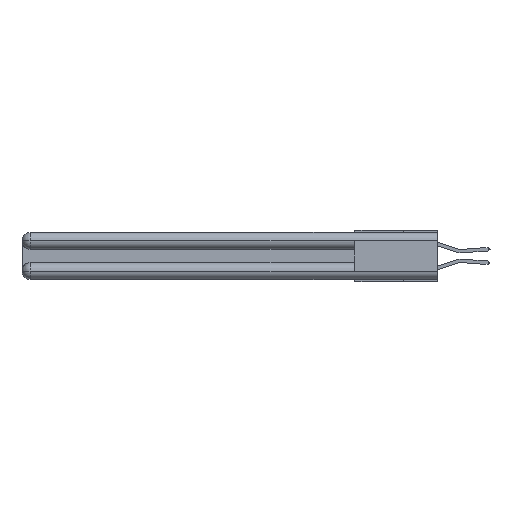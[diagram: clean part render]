
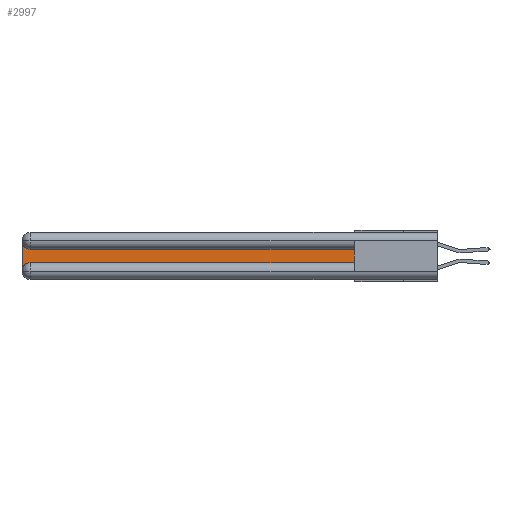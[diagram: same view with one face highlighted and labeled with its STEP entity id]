
A CAD part, left-side view. The second image highlights one B-rep face of the part: STEP entity #2997.
In plain terms, the highlighted planar face has unit normal (-1, 0, 0).
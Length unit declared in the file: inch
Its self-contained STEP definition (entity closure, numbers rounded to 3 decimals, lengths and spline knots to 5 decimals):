
#1383 = CARTESIAN_POINT ( 'NONE',  ( 0.075, 3., -0.1225 ) ) ;
#1906 = EDGE_CURVE ( 'NONE', #7431, #24839, #16545, .T. ) ;
#2241 = CARTESIAN_POINT ( 'NONE',  ( 0.075, 0.6, -0.2175 ) ) ;
#2537 = FACE_OUTER_BOUND ( 'NONE', #21836, .T. ) ;
#2909 = DIRECTION ( 'NONE',  ( 0., 0., 1. ) ) ;
#2997 = ADVANCED_FACE ( 'NONE', ( #2537 ), #21631, .F. ) ;
#3498 = CARTESIAN_POINT ( 'NONE',  ( 0.075, 3., -0.2175 ) ) ;
#3746 = VERTEX_POINT ( 'NONE', #27818 ) ;
#3760 = AXIS2_PLACEMENT_3D ( 'NONE', #4297, #11022, #17726 ) ;
#3941 = EDGE_CURVE ( 'NONE', #19780, #12623, #18154, .T. ) ;
#4297 = CARTESIAN_POINT ( 'NONE',  ( 0.075, 2.94, -0.0625 ) ) ;
#5519 = AXIS2_PLACEMENT_3D ( 'NONE', #1383, #22211, #5997 ) ;
#5698 = LINE ( 'NONE', #8491, #6727 ) ;
#5997 = DIRECTION ( 'NONE',  ( 0., 0., -1. ) ) ;
#6366 = ORIENTED_EDGE ( 'NONE', *, *, #25908, .T. ) ;
#6727 = VECTOR ( 'NONE', #8200, 39.37008 ) ;
#6818 = DIRECTION ( 'NONE',  ( 0., 0., -1. ) ) ;
#7431 = VERTEX_POINT ( 'NONE', #28076 ) ;
#8200 = DIRECTION ( 'NONE',  ( 0., 1., 0. ) ) ;
#8491 = CARTESIAN_POINT ( 'NONE',  ( 0.075, 0.6, -0.1225 ) ) ;
#10344 = DIRECTION ( 'NONE',  ( 0., 0., -1. ) ) ;
#10437 = EDGE_CURVE ( 'NONE', #16389, #19780, #12379, .T. ) ;
#10933 = EDGE_CURVE ( 'NONE', #12623, #7431, #21780, .T. ) ;
#11022 = DIRECTION ( 'NONE',  ( 1., 0., 0. ) ) ;
#12379 = LINE ( 'NONE', #3498, #27398 ) ;
#12623 = VERTEX_POINT ( 'NONE', #16367 ) ;
#13948 = ORIENTED_EDGE ( 'NONE', *, *, #21478, .T. ) ;
#15793 = DIRECTION ( 'NONE',  ( 1., 0., 0. ) ) ;
#15933 = ORIENTED_EDGE ( 'NONE', *, *, #10437, .T. ) ;
#16367 = CARTESIAN_POINT ( 'NONE',  ( 0.075, 2.94, -0.2175 ) ) ;
#16389 = VERTEX_POINT ( 'NONE', #24793 ) ;
#16545 = LINE ( 'NONE', #23099, #18955 ) ;
#17726 = DIRECTION ( 'NONE',  ( 0., 0., -1. ) ) ;
#18154 = CIRCLE ( 'NONE', #22731, 0.06 ) ;
#18955 = VECTOR ( 'NONE', #2909, 39.37008 ) ;
#19367 = CIRCLE ( 'NONE', #3760, 0.06 ) ;
#19737 = ORIENTED_EDGE ( 'NONE', *, *, #10933, .T. ) ;
#19780 = VERTEX_POINT ( 'NONE', #23600 ) ;
#21478 = EDGE_CURVE ( 'NONE', #24839, #3746, #5698, .T. ) ;
#21631 = PLANE ( 'NONE',  #5519 ) ;
#21780 = LINE ( 'NONE', #2241, #28414 ) ;
#21836 = EDGE_LOOP ( 'NONE', ( #13948, #6366, #15933, #24342, #19737, #22101 ) ) ;
#21841 = DIRECTION ( 'NONE',  ( 0., -1., 0. ) ) ;
#22101 = ORIENTED_EDGE ( 'NONE', *, *, #1906, .T. ) ;
#22211 = DIRECTION ( 'NONE',  ( 1., 0., 0. ) ) ;
#22225 = CARTESIAN_POINT ( 'NONE',  ( 0.075, 2.94, -0.2775 ) ) ;
#22731 = AXIS2_PLACEMENT_3D ( 'NONE', #22225, #15793, #6818 ) ;
#23099 = CARTESIAN_POINT ( 'NONE',  ( 0.075, 0.6, -0.2175 ) ) ;
#23600 = CARTESIAN_POINT ( 'NONE',  ( 0.075, 3., -0.2775 ) ) ;
#23800 = CARTESIAN_POINT ( 'NONE',  ( 0.075, 0.6, -0.1225 ) ) ;
#24342 = ORIENTED_EDGE ( 'NONE', *, *, #3941, .T. ) ;
#24793 = CARTESIAN_POINT ( 'NONE',  ( 0.075, 3., -0.0625 ) ) ;
#24839 = VERTEX_POINT ( 'NONE', #23800 ) ;
#25908 = EDGE_CURVE ( 'NONE', #3746, #16389, #19367, .T. ) ;
#27398 = VECTOR ( 'NONE', #10344, 39.37008 ) ;
#27818 = CARTESIAN_POINT ( 'NONE',  ( 0.075, 2.94, -0.1225 ) ) ;
#28076 = CARTESIAN_POINT ( 'NONE',  ( 0.075, 0.6, -0.2175 ) ) ;
#28414 = VECTOR ( 'NONE', #21841, 39.37008 ) ;
